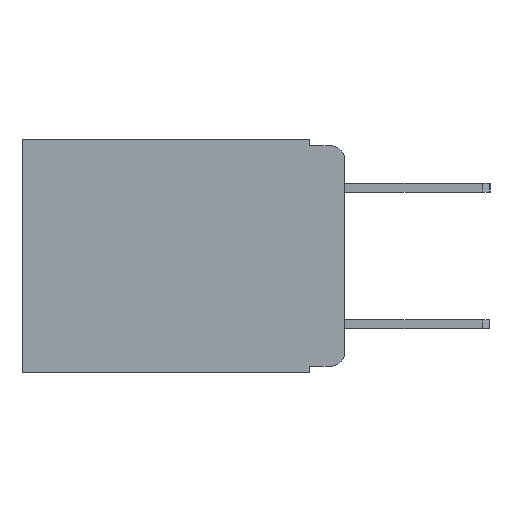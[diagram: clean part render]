
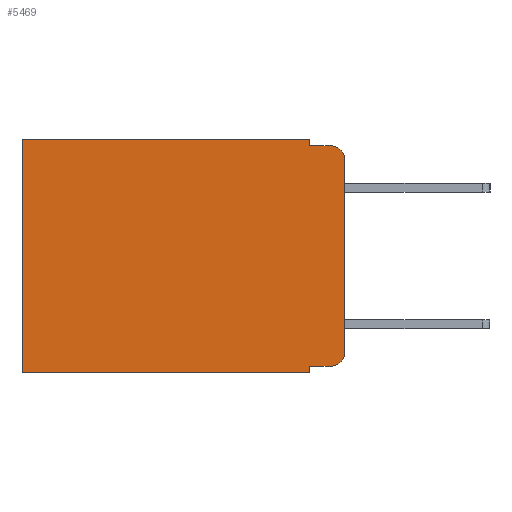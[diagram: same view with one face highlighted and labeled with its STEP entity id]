
A CAD part, left-side view. The second image highlights one B-rep face of the part: STEP entity #5469.
In plain terms, the highlighted planar face has unit normal (-1, 0, 0).
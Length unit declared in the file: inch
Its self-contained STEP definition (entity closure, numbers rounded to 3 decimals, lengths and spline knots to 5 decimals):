
#68 = CARTESIAN_POINT ( 'NONE',  ( 0.298, 0., 0. ) ) ;
#94 = CARTESIAN_POINT ( 'NONE',  ( 0.298, 0.051, -0.343 ) ) ;
#580 = CARTESIAN_POINT ( 'NONE',  ( 0.298, 0.473, 0. ) ) ;
#972 = EDGE_CURVE ( 'NONE', #10011, #10506, #13460, .T. ) ;
#1443 = CARTESIAN_POINT ( 'NONE',  ( 0.298, 0.051, -0.333 ) ) ;
#1460 = ORIENTED_EDGE ( 'NONE', *, *, #972, .T. ) ;
#1499 = EDGE_CURVE ( 'NONE', #8254, #4348, #5052, .T. ) ;
#2185 = CARTESIAN_POINT ( 'NONE',  ( 0.298, 0., -0.03 ) ) ;
#3018 = DIRECTION ( 'NONE',  ( 0., 0., -1. ) ) ;
#3277 = EDGE_CURVE ( 'NONE', #10011, #8254, #14835, .T. ) ;
#3705 = LINE ( 'NONE', #13122, #18803 ) ;
#3749 = DIRECTION ( 'NONE',  ( 0., 1., 0. ) ) ;
#3866 = CARTESIAN_POINT ( 'NONE',  ( 0.298, 0.473, -0.343 ) ) ;
#4279 = ORIENTED_EDGE ( 'NONE', *, *, #18893, .T. ) ;
#4348 = VERTEX_POINT ( 'NONE', #3866 ) ;
#4371 = EDGE_CURVE ( 'NONE', #10675, #4348, #11117, .T. ) ;
#5052 = LINE ( 'NONE', #17728, #16398 ) ;
#5236 = DIRECTION ( 'NONE',  ( 0., -1., 0. ) ) ;
#5460 = EDGE_CURVE ( 'NONE', #8848, #9850, #17408, .T. ) ;
#5469 = ADVANCED_FACE ( 'NONE', ( #6297 ), #17097, .F. ) ;
#5684 = DIRECTION ( 'NONE',  ( -1., 0., 0. ) ) ;
#5717 = CARTESIAN_POINT ( 'NONE',  ( 0.298, 0.051, -0.333 ) ) ;
#5889 = AXIS2_PLACEMENT_3D ( 'NONE', #13039, #18410, #10364 ) ;
#6039 = DIRECTION ( 'NONE',  ( -1., 0., 0. ) ) ;
#6061 = ORIENTED_EDGE ( 'NONE', *, *, #3277, .F. ) ;
#6297 = FACE_OUTER_BOUND ( 'NONE', #6357, .T. ) ;
#6308 = AXIS2_PLACEMENT_3D ( 'NONE', #14222, #5684, #15619 ) ;
#6357 = EDGE_LOOP ( 'NONE', ( #10001, #12081, #12617, #12884, #13435, #13512, #8028, #6061, #1460, #4279 ) ) ;
#6525 = EDGE_CURVE ( 'NONE', #9850, #14892, #3705, .T. ) ;
#6976 = DIRECTION ( 'NONE',  ( 0., 1., 0. ) ) ;
#7276 = VECTOR ( 'NONE', #9654, 39.37008 ) ;
#7295 = DIRECTION ( 'NONE',  ( 0., 0., -1. ) ) ;
#7583 = VERTEX_POINT ( 'NONE', #2185 ) ;
#7721 = CARTESIAN_POINT ( 'NONE',  ( 0.298, 0.02, -0.01 ) ) ;
#7738 = VECTOR ( 'NONE', #11482, 39.37008 ) ;
#7911 = CARTESIAN_POINT ( 'NONE',  ( 0.298, 0.02, -0.333 ) ) ;
#8028 = ORIENTED_EDGE ( 'NONE', *, *, #1499, .F. ) ;
#8062 = CIRCLE ( 'NONE', #6308, 0.02 ) ;
#8254 = VERTEX_POINT ( 'NONE', #94 ) ;
#8412 = CIRCLE ( 'NONE', #16440, 0.02 ) ;
#8502 = EDGE_CURVE ( 'NONE', #7583, #14892, #8062, .T. ) ;
#8848 = VERTEX_POINT ( 'NONE', #14764 ) ;
#9654 = DIRECTION ( 'NONE',  ( 0., 0., -1. ) ) ;
#9850 = VERTEX_POINT ( 'NONE', #17982 ) ;
#10001 = ORIENTED_EDGE ( 'NONE', *, *, #15944, .F. ) ;
#10011 = VERTEX_POINT ( 'NONE', #5717 ) ;
#10099 = LINE ( 'NONE', #11268, #16483 ) ;
#10214 = VECTOR ( 'NONE', #7295, 39.37008 ) ;
#10364 = DIRECTION ( 'NONE',  ( 0., 0., -1. ) ) ;
#10506 = VERTEX_POINT ( 'NONE', #7911 ) ;
#10675 = VERTEX_POINT ( 'NONE', #11110 ) ;
#10803 = VECTOR ( 'NONE', #3018, 39.37008 ) ;
#11110 = CARTESIAN_POINT ( 'NONE',  ( 0.298, 0.473, 0. ) ) ;
#11116 = LINE ( 'NONE', #68, #7276 ) ;
#11117 = LINE ( 'NONE', #580, #7738 ) ;
#11268 = CARTESIAN_POINT ( 'NONE',  ( 0.298, 0., 0. ) ) ;
#11482 = DIRECTION ( 'NONE',  ( 0., 0., -1. ) ) ;
#11595 = CARTESIAN_POINT ( 'NONE',  ( 0.298, 0., -0.313 ) ) ;
#12081 = ORIENTED_EDGE ( 'NONE', *, *, #8502, .T. ) ;
#12596 = VECTOR ( 'NONE', #5236, 39.37008 ) ;
#12617 = ORIENTED_EDGE ( 'NONE', *, *, #6525, .F. ) ;
#12884 = ORIENTED_EDGE ( 'NONE', *, *, #5460, .F. ) ;
#13039 = CARTESIAN_POINT ( 'NONE',  ( 0.298, 0., 0. ) ) ;
#13122 = CARTESIAN_POINT ( 'NONE',  ( 0.298, 0.051, -0.01 ) ) ;
#13381 = CARTESIAN_POINT ( 'NONE',  ( 0.298, 0.051, 0. ) ) ;
#13435 = ORIENTED_EDGE ( 'NONE', *, *, #14004, .T. ) ;
#13460 = LINE ( 'NONE', #1443, #12596 ) ;
#13512 = ORIENTED_EDGE ( 'NONE', *, *, #4371, .T. ) ;
#14004 = EDGE_CURVE ( 'NONE', #8848, #10675, #10099, .T. ) ;
#14222 = CARTESIAN_POINT ( 'NONE',  ( 0.298, 0.02, -0.03 ) ) ;
#14465 = DIRECTION ( 'NONE',  ( 0., -1., 0. ) ) ;
#14507 = CARTESIAN_POINT ( 'NONE',  ( 0.298, 0.02, -0.313 ) ) ;
#14764 = CARTESIAN_POINT ( 'NONE',  ( 0.298, 0.051, 0. ) ) ;
#14835 = LINE ( 'NONE', #13381, #10803 ) ;
#14892 = VERTEX_POINT ( 'NONE', #7721 ) ;
#15619 = DIRECTION ( 'NONE',  ( 0., 0., -1. ) ) ;
#15915 = DIRECTION ( 'NONE',  ( 0., 0., -1. ) ) ;
#15944 = EDGE_CURVE ( 'NONE', #7583, #17071, #11116, .T. ) ;
#16398 = VECTOR ( 'NONE', #6976, 39.37008 ) ;
#16440 = AXIS2_PLACEMENT_3D ( 'NONE', #14507, #6039, #15915 ) ;
#16483 = VECTOR ( 'NONE', #3749, 39.37008 ) ;
#17071 = VERTEX_POINT ( 'NONE', #11595 ) ;
#17097 = PLANE ( 'NONE',  #5889 ) ;
#17408 = LINE ( 'NONE', #18353, #10214 ) ;
#17728 = CARTESIAN_POINT ( 'NONE',  ( 0.298, 0., -0.343 ) ) ;
#17982 = CARTESIAN_POINT ( 'NONE',  ( 0.298, 0.051, -0.01 ) ) ;
#18353 = CARTESIAN_POINT ( 'NONE',  ( 0.298, 0.051, 0. ) ) ;
#18410 = DIRECTION ( 'NONE',  ( 1., 0., 0. ) ) ;
#18803 = VECTOR ( 'NONE', #14465, 39.37008 ) ;
#18893 = EDGE_CURVE ( 'NONE', #10506, #17071, #8412, .T. ) ;
